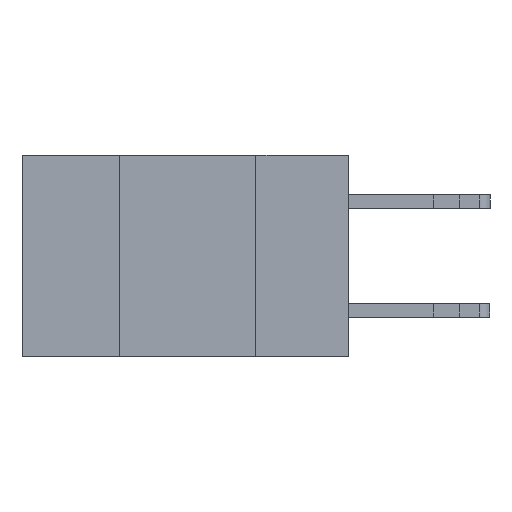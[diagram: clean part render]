
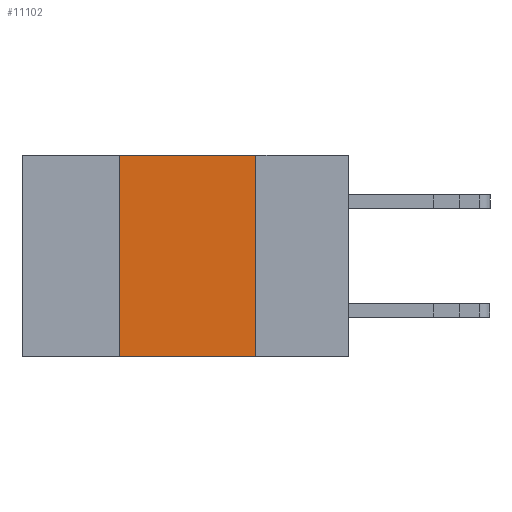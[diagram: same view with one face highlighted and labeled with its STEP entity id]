
A CAD part, left-side view. The second image highlights one B-rep face of the part: STEP entity #11102.
In plain terms, the highlighted planar face has unit normal (-1, 0, 0).
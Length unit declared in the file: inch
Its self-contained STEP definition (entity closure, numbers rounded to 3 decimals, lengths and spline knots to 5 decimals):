
#1197 = ORIENTED_EDGE ( 'NONE', *, *, #10191, .F. ) ;
#1524 = ORIENTED_EDGE ( 'NONE', *, *, #23828, .F. ) ;
#1699 = DIRECTION ( 'NONE',  ( 0., 0., -1. ) ) ;
#2631 = CARTESIAN_POINT ( 'NONE',  ( 0., 0.6, 0. ) ) ;
#2645 = EDGE_LOOP ( 'NONE', ( #1524, #1197, #26983, #4228 ) ) ;
#3676 = FACE_OUTER_BOUND ( 'NONE', #2645, .T. ) ;
#3948 = VECTOR ( 'NONE', #14977, 39.37008 ) ;
#4228 = ORIENTED_EDGE ( 'NONE', *, *, #12588, .T. ) ;
#10191 = EDGE_CURVE ( 'NONE', #15504, #17872, #22852, .T. ) ;
#10291 = DIRECTION ( 'NONE',  ( 0., -1., 0. ) ) ;
#11102 = ADVANCED_FACE ( 'NONE', ( #3676 ), #12263, .F. ) ;
#11270 = LINE ( 'NONE', #25443, #16169 ) ;
#11480 = VERTEX_POINT ( 'NONE', #19733 ) ;
#12263 = PLANE ( 'NONE',  #13037 ) ;
#12588 = EDGE_CURVE ( 'NONE', #23715, #11480, #11270, .T. ) ;
#12886 = CARTESIAN_POINT ( 'NONE',  ( 0., 0.17, 0. ) ) ;
#13037 = AXIS2_PLACEMENT_3D ( 'NONE', #26995, #14340, #1699 ) ;
#14340 = DIRECTION ( 'NONE',  ( 1., 0., 0. ) ) ;
#14502 = LINE ( 'NONE', #12886, #3948 ) ;
#14617 = CARTESIAN_POINT ( 'NONE',  ( 0., 0.42, -0.37 ) ) ;
#14977 = DIRECTION ( 'NONE',  ( 0., 0., -1. ) ) ;
#15504 = VERTEX_POINT ( 'NONE', #22478 ) ;
#16169 = VECTOR ( 'NONE', #10291, 39.37008 ) ;
#17288 = VECTOR ( 'NONE', #21558, 39.37008 ) ;
#17872 = VERTEX_POINT ( 'NONE', #22947 ) ;
#18907 = LINE ( 'NONE', #21921, #24547 ) ;
#19583 = EDGE_CURVE ( 'NONE', #23715, #15504, #18907, .T. ) ;
#19733 = CARTESIAN_POINT ( 'NONE',  ( 0., 0.17, -0.37 ) ) ;
#21558 = DIRECTION ( 'NONE',  ( 0., -1., 0. ) ) ;
#21921 = CARTESIAN_POINT ( 'NONE',  ( 0., 0.42, 0. ) ) ;
#22478 = CARTESIAN_POINT ( 'NONE',  ( 0., 0.42, 0. ) ) ;
#22852 = LINE ( 'NONE', #2631, #17288 ) ;
#22947 = CARTESIAN_POINT ( 'NONE',  ( 0., 0.17, 0. ) ) ;
#23715 = VERTEX_POINT ( 'NONE', #14617 ) ;
#23828 = EDGE_CURVE ( 'NONE', #17872, #11480, #14502, .T. ) ;
#24104 = DIRECTION ( 'NONE',  ( 0., 0., 1. ) ) ;
#24547 = VECTOR ( 'NONE', #24104, 39.37008 ) ;
#25443 = CARTESIAN_POINT ( 'NONE',  ( 0., 0.6, -0.37 ) ) ;
#26983 = ORIENTED_EDGE ( 'NONE', *, *, #19583, .F. ) ;
#26995 = CARTESIAN_POINT ( 'NONE',  ( 0., 0.6, 0. ) ) ;
